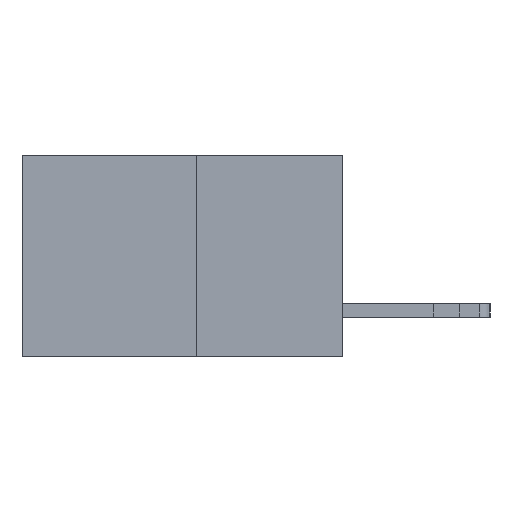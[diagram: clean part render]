
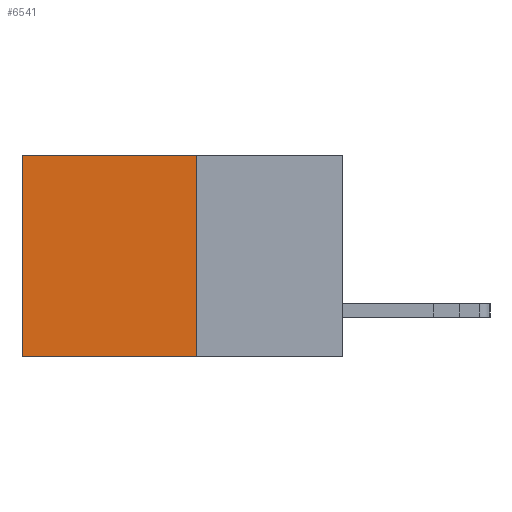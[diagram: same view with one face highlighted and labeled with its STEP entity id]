
A CAD part, left-side view. The second image highlights one B-rep face of the part: STEP entity #6541.
In plain terms, the highlighted planar face has unit normal (-1, 0, 0).
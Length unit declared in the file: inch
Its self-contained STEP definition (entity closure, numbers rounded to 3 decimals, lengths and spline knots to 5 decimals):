
#210 = VECTOR ( 'NONE', #2160, 39.37008 ) ;
#875 = DIRECTION ( 'NONE',  ( 0., 1., 0. ) ) ;
#1529 = CARTESIAN_POINT ( 'NONE',  ( 0.277, 0.27, -0.37 ) ) ;
#2096 = CARTESIAN_POINT ( 'NONE',  ( 0.277, 0.27, 0. ) ) ;
#2160 = DIRECTION ( 'NONE',  ( 0., 1., 0. ) ) ;
#3524 = CARTESIAN_POINT ( 'NONE',  ( 0.277, 0.27, -0.37 ) ) ;
#4279 = CARTESIAN_POINT ( 'NONE',  ( 0.277, 0.59, -0.37 ) ) ;
#4348 = LINE ( 'NONE', #6053, #12780 ) ;
#4591 = AXIS2_PLACEMENT_3D ( 'NONE', #1529, #20166, #9936 ) ;
#4757 = ORIENTED_EDGE ( 'NONE', *, *, #8690, .F. ) ;
#5433 = FACE_OUTER_BOUND ( 'NONE', #10605, .T. ) ;
#5449 = CARTESIAN_POINT ( 'NONE',  ( 0.277, 0.27, 0. ) ) ;
#5980 = DIRECTION ( 'NONE',  ( 0., 0., -1. ) ) ;
#6053 = CARTESIAN_POINT ( 'NONE',  ( 0.277, 0.27, -0.37 ) ) ;
#6541 = ADVANCED_FACE ( 'NONE', ( #5433 ), #8247, .F. ) ;
#6662 = LINE ( 'NONE', #3524, #14669 ) ;
#6801 = EDGE_CURVE ( 'NONE', #8245, #20887, #13612, .T. ) ;
#6871 = LINE ( 'NONE', #4279, #15414 ) ;
#7031 = EDGE_CURVE ( 'NONE', #16175, #17735, #4348, .T. ) ;
#7319 = CARTESIAN_POINT ( 'NONE',  ( 0.277, 0.59, 0. ) ) ;
#7805 = ORIENTED_EDGE ( 'NONE', *, *, #7031, .F. ) ;
#8245 = VERTEX_POINT ( 'NONE', #5449 ) ;
#8247 = PLANE ( 'NONE',  #4591 ) ;
#8634 = CARTESIAN_POINT ( 'NONE',  ( 0.277, 0.27, -0.37 ) ) ;
#8690 = EDGE_CURVE ( 'NONE', #8245, #16175, #6662, .T. ) ;
#8742 = ORIENTED_EDGE ( 'NONE', *, *, #9684, .T. ) ;
#9684 = EDGE_CURVE ( 'NONE', #20887, #17735, #6871, .T. ) ;
#9936 = DIRECTION ( 'NONE',  ( 0., 0., -1. ) ) ;
#10605 = EDGE_LOOP ( 'NONE', ( #8742, #7805, #4757, #13931 ) ) ;
#12780 = VECTOR ( 'NONE', #875, 39.37008 ) ;
#13612 = LINE ( 'NONE', #2096, #210 ) ;
#13631 = DIRECTION ( 'NONE',  ( 0., 0., -1. ) ) ;
#13931 = ORIENTED_EDGE ( 'NONE', *, *, #6801, .T. ) ;
#14669 = VECTOR ( 'NONE', #13631, 39.37008 ) ;
#15414 = VECTOR ( 'NONE', #5980, 39.37008 ) ;
#16175 = VERTEX_POINT ( 'NONE', #8634 ) ;
#17735 = VERTEX_POINT ( 'NONE', #20621 ) ;
#20166 = DIRECTION ( 'NONE',  ( 1., 0., 0. ) ) ;
#20621 = CARTESIAN_POINT ( 'NONE',  ( 0.277, 0.59, -0.37 ) ) ;
#20887 = VERTEX_POINT ( 'NONE', #7319 ) ;
